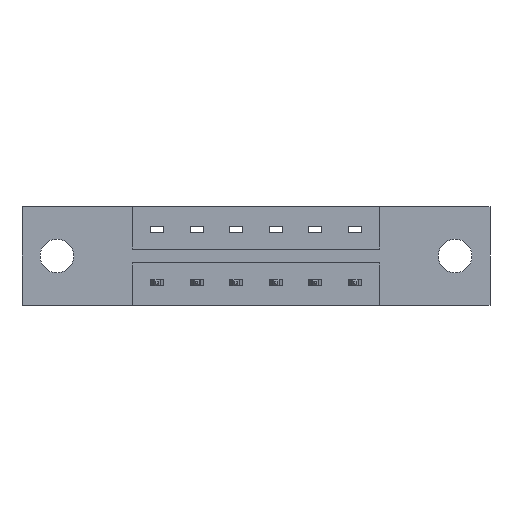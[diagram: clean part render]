
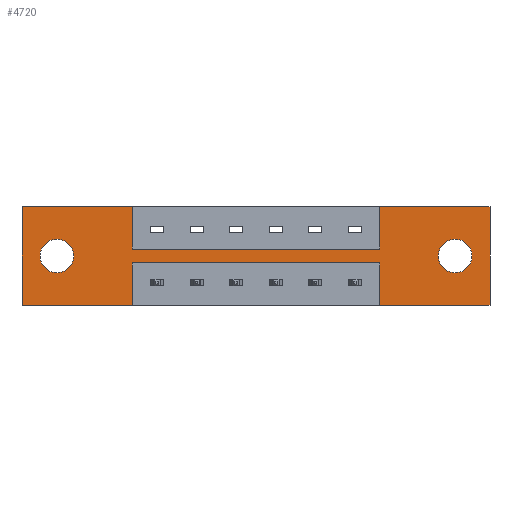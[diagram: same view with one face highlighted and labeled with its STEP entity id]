
A CAD part, front view. The second image highlights one B-rep face of the part: STEP entity #4720.
In plain terms, the highlighted planar face has unit normal (0, -1, 0).
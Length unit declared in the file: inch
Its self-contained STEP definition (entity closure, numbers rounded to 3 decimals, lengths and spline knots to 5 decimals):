
#126 = VERTEX_POINT ( 'NONE', #2826 ) ;
#157 = LINE ( 'NONE', #3902, #3286 ) ;
#171 = VECTOR ( 'NONE', #5851, 39.37008 ) ;
#455 = VECTOR ( 'NONE', #1524, 39.37008 ) ;
#487 = VERTEX_POINT ( 'NONE', #7712 ) ;
#570 = VECTOR ( 'NONE', #8237, 39.37008 ) ;
#605 = EDGE_CURVE ( 'NONE', #5778, #6451, #2992, .T. ) ;
#621 = CARTESIAN_POINT ( 'NONE',  ( 1.6425, 0., -0.2515 ) ) ;
#674 = ORIENTED_EDGE ( 'NONE', *, *, #7294, .F. ) ;
#721 = EDGE_CURVE ( 'NONE', #6205, #6852, #7734, .T. ) ;
#841 = EDGE_LOOP ( 'NONE', ( #1278, #674, #7091, #7510, #3355, #1827, #4442, #4466, #1448, #4593, #5694, #3701 ) ) ;
#894 = CARTESIAN_POINT ( 'NONE',  ( 0.4175, 0., -0.214 ) ) ;
#957 = EDGE_LOOP ( 'NONE', ( #3068, #5114 ) ) ;
#968 = CIRCLE ( 'NONE', #5069, 0.064 ) ;
#1029 = DIRECTION ( 'NONE',  ( 0., 1., 0. ) ) ;
#1107 = CARTESIAN_POINT ( 'NONE',  ( 0., 0., 0. ) ) ;
#1278 = ORIENTED_EDGE ( 'NONE', *, *, #4836, .F. ) ;
#1393 = EDGE_CURVE ( 'NONE', #1395, #4899, #5000, .T. ) ;
#1395 = VERTEX_POINT ( 'NONE', #6975 ) ;
#1448 = ORIENTED_EDGE ( 'NONE', *, *, #605, .F. ) ;
#1524 = DIRECTION ( 'NONE',  ( 0., 0., -1. ) ) ;
#1671 = LINE ( 'NONE', #2417, #5581 ) ;
#1817 = EDGE_CURVE ( 'NONE', #5523, #2225, #3481, .T. ) ;
#1827 = ORIENTED_EDGE ( 'NONE', *, *, #7455, .F. ) ;
#1871 = LINE ( 'NONE', #5779, #5684 ) ;
#1901 = EDGE_CURVE ( 'NONE', #2188, #126, #1984, .T. ) ;
#1923 = DIRECTION ( 'NONE',  ( 0., 0., -1. ) ) ;
#1935 = AXIS2_PLACEMENT_3D ( 'NONE', #4803, #6666, #2813 ) ;
#1984 = LINE ( 'NONE', #894, #455 ) ;
#2065 = CARTESIAN_POINT ( 'NONE',  ( 0.1325, 0., -0.2515 ) ) ;
#2150 = VERTEX_POINT ( 'NONE', #5043 ) ;
#2188 = VERTEX_POINT ( 'NONE', #6986 ) ;
#2211 = LINE ( 'NONE', #7557, #3015 ) ;
#2221 = CARTESIAN_POINT ( 'NONE',  ( 0.4175, 0., -0.161 ) ) ;
#2224 = CARTESIAN_POINT ( 'NONE',  ( 0.1325, 0., -0.1875 ) ) ;
#2225 = VERTEX_POINT ( 'NONE', #621 ) ;
#2317 = CARTESIAN_POINT ( 'NONE',  ( 0., 0., -0.375 ) ) ;
#2417 = CARTESIAN_POINT ( 'NONE',  ( 0.4175, 0., -0.214 ) ) ;
#2535 = AXIS2_PLACEMENT_3D ( 'NONE', #2224, #6041, #4019 ) ;
#2573 = VECTOR ( 'NONE', #5951, 39.37008 ) ;
#2580 = CARTESIAN_POINT ( 'NONE',  ( 0., 0., 0. ) ) ;
#2626 = LINE ( 'NONE', #5104, #5155 ) ;
#2667 = CARTESIAN_POINT ( 'NONE',  ( 1.3575, 0., -0.214 ) ) ;
#2702 = EDGE_CURVE ( 'NONE', #5014, #1395, #4282, .T. ) ;
#2813 = DIRECTION ( 'NONE',  ( 0., 0., -1. ) ) ;
#2826 = CARTESIAN_POINT ( 'NONE',  ( 0.4175, 0., -0.375 ) ) ;
#2886 = VECTOR ( 'NONE', #4833, 39.37008 ) ;
#2893 = CARTESIAN_POINT ( 'NONE',  ( 0.4175, 0., -0.161 ) ) ;
#2992 = LINE ( 'NONE', #4559, #171 ) ;
#3015 = VECTOR ( 'NONE', #3689, 39.37008 ) ;
#3050 = DIRECTION ( 'NONE',  ( -1., 0., 0. ) ) ;
#3068 = ORIENTED_EDGE ( 'NONE', *, *, #7592, .T. ) ;
#3094 = EDGE_CURVE ( 'NONE', #487, #4191, #6080, .T. ) ;
#3184 = DIRECTION ( 'NONE',  ( 0., 1., 0. ) ) ;
#3195 = ORIENTED_EDGE ( 'NONE', *, *, #1817, .T. ) ;
#3244 = CARTESIAN_POINT ( 'NONE',  ( 0.4175, 0., -0.161 ) ) ;
#3286 = VECTOR ( 'NONE', #6563, 39.37008 ) ;
#3355 = ORIENTED_EDGE ( 'NONE', *, *, #2702, .F. ) ;
#3417 = CARTESIAN_POINT ( 'NONE',  ( 1.3575, 0., -0.161 ) ) ;
#3471 = ORIENTED_EDGE ( 'NONE', *, *, #5888, .T. ) ;
#3481 = CIRCLE ( 'NONE', #1935, 0.064 ) ;
#3689 = DIRECTION ( 'NONE',  ( 0., 0., -1. ) ) ;
#3701 = ORIENTED_EDGE ( 'NONE', *, *, #7673, .F. ) ;
#3710 = AXIS2_PLACEMENT_3D ( 'NONE', #4911, #3184, #1923 ) ;
#3902 = CARTESIAN_POINT ( 'NONE',  ( 0., 0., -0.375 ) ) ;
#3934 = FACE_BOUND ( 'NONE', #957, .T. ) ;
#3955 = DIRECTION ( 'NONE',  ( -1., 0., 0. ) ) ;
#4019 = DIRECTION ( 'NONE',  ( 0., 0., 1. ) ) ;
#4191 = VERTEX_POINT ( 'NONE', #2221 ) ;
#4211 = CARTESIAN_POINT ( 'NONE',  ( 1.3575, 0., -0.375 ) ) ;
#4249 = DIRECTION ( 'NONE',  ( 0., -1., 0. ) ) ;
#4282 = LINE ( 'NONE', #3417, #2573 ) ;
#4351 = AXIS2_PLACEMENT_3D ( 'NONE', #2317, #4249, #8042 ) ;
#4366 = VECTOR ( 'NONE', #5685, 39.37008 ) ;
#4442 = ORIENTED_EDGE ( 'NONE', *, *, #3094, .F. ) ;
#4466 = ORIENTED_EDGE ( 'NONE', *, *, #4552, .F. ) ;
#4474 = DIRECTION ( 'NONE',  ( 0., 0., 1. ) ) ;
#4491 = LINE ( 'NONE', #2893, #2886 ) ;
#4521 = DIRECTION ( 'NONE',  ( 1., 0., 0. ) ) ;
#4552 = EDGE_CURVE ( 'NONE', #6451, #487, #7366, .T. ) ;
#4559 = CARTESIAN_POINT ( 'NONE',  ( 0., 0., 0. ) ) ;
#4593 = ORIENTED_EDGE ( 'NONE', *, *, #7313, .F. ) ;
#4706 = CARTESIAN_POINT ( 'NONE',  ( 0.1325, 0., -0.1235 ) ) ;
#4720 = ADVANCED_FACE ( 'NONE', ( #7069, #3934, #5359 ), #6132, .T. ) ;
#4727 = CARTESIAN_POINT ( 'NONE',  ( 1.6425, 0., -0.1235 ) ) ;
#4803 = CARTESIAN_POINT ( 'NONE',  ( 1.6425, 0., -0.1875 ) ) ;
#4833 = DIRECTION ( 'NONE',  ( 1., 0., 0. ) ) ;
#4836 = EDGE_CURVE ( 'NONE', #5768, #5450, #2626, .T. ) ;
#4899 = VERTEX_POINT ( 'NONE', #5167 ) ;
#4911 = CARTESIAN_POINT ( 'NONE',  ( 1.6425, 0., -0.1875 ) ) ;
#5000 = LINE ( 'NONE', #7517, #570 ) ;
#5014 = VERTEX_POINT ( 'NONE', #7264 ) ;
#5043 = CARTESIAN_POINT ( 'NONE',  ( 1.775, 0., -0.375 ) ) ;
#5069 = AXIS2_PLACEMENT_3D ( 'NONE', #6210, #1029, #6867 ) ;
#5104 = CARTESIAN_POINT ( 'NONE',  ( 1.3575, 0., -0.214 ) ) ;
#5114 = ORIENTED_EDGE ( 'NONE', *, *, #721, .T. ) ;
#5155 = VECTOR ( 'NONE', #4474, 39.37008 ) ;
#5167 = CARTESIAN_POINT ( 'NONE',  ( 1.775, 0., 0. ) ) ;
#5359 = FACE_OUTER_BOUND ( 'NONE', #841, .T. ) ;
#5450 = VERTEX_POINT ( 'NONE', #2667 ) ;
#5523 = VERTEX_POINT ( 'NONE', #4727 ) ;
#5581 = VECTOR ( 'NONE', #3050, 39.37008 ) ;
#5684 = VECTOR ( 'NONE', #3955, 39.37008 ) ;
#5685 = DIRECTION ( 'NONE',  ( 0., 0., -1. ) ) ;
#5694 = ORIENTED_EDGE ( 'NONE', *, *, #1901, .F. ) ;
#5768 = VERTEX_POINT ( 'NONE', #4211 ) ;
#5778 = VERTEX_POINT ( 'NONE', #7452 ) ;
#5779 = CARTESIAN_POINT ( 'NONE',  ( 0., 0., -0.375 ) ) ;
#5784 = EDGE_CURVE ( 'NONE', #4899, #2150, #2211, .T. ) ;
#5851 = DIRECTION ( 'NONE',  ( 0., 0., 1. ) ) ;
#5888 = EDGE_CURVE ( 'NONE', #2225, #5523, #7146, .T. ) ;
#5951 = DIRECTION ( 'NONE',  ( 0., 0., 1. ) ) ;
#6041 = DIRECTION ( 'NONE',  ( 0., 1., 0. ) ) ;
#6080 = LINE ( 'NONE', #3244, #4366 ) ;
#6132 = PLANE ( 'NONE',  #4351 ) ;
#6205 = VERTEX_POINT ( 'NONE', #2065 ) ;
#6210 = CARTESIAN_POINT ( 'NONE',  ( 0.1325, 0., -0.1875 ) ) ;
#6451 = VERTEX_POINT ( 'NONE', #1107 ) ;
#6563 = DIRECTION ( 'NONE',  ( -1., 0., 0. ) ) ;
#6666 = DIRECTION ( 'NONE',  ( 0., 1., 0. ) ) ;
#6668 = VECTOR ( 'NONE', #4521, 39.37008 ) ;
#6852 = VERTEX_POINT ( 'NONE', #4706 ) ;
#6867 = DIRECTION ( 'NONE',  ( 0., 0., 1. ) ) ;
#6880 = EDGE_LOOP ( 'NONE', ( #3195, #3471 ) ) ;
#6975 = CARTESIAN_POINT ( 'NONE',  ( 1.3575, 0., 0. ) ) ;
#6986 = CARTESIAN_POINT ( 'NONE',  ( 0.4175, 0., -0.214 ) ) ;
#7069 = FACE_BOUND ( 'NONE', #6880, .T. ) ;
#7091 = ORIENTED_EDGE ( 'NONE', *, *, #5784, .F. ) ;
#7146 = CIRCLE ( 'NONE', #3710, 0.064 ) ;
#7264 = CARTESIAN_POINT ( 'NONE',  ( 1.3575, 0., -0.161 ) ) ;
#7294 = EDGE_CURVE ( 'NONE', #2150, #5768, #157, .T. ) ;
#7313 = EDGE_CURVE ( 'NONE', #126, #5778, #1871, .T. ) ;
#7366 = LINE ( 'NONE', #2580, #6668 ) ;
#7452 = CARTESIAN_POINT ( 'NONE',  ( 0., 0., -0.375 ) ) ;
#7455 = EDGE_CURVE ( 'NONE', #4191, #5014, #4491, .T. ) ;
#7510 = ORIENTED_EDGE ( 'NONE', *, *, #1393, .F. ) ;
#7517 = CARTESIAN_POINT ( 'NONE',  ( 0., 0., 0. ) ) ;
#7557 = CARTESIAN_POINT ( 'NONE',  ( 1.775, 0., 0. ) ) ;
#7592 = EDGE_CURVE ( 'NONE', #6852, #6205, #968, .T. ) ;
#7673 = EDGE_CURVE ( 'NONE', #5450, #2188, #1671, .T. ) ;
#7712 = CARTESIAN_POINT ( 'NONE',  ( 0.4175, 0., 0. ) ) ;
#7734 = CIRCLE ( 'NONE', #2535, 0.064 ) ;
#8042 = DIRECTION ( 'NONE',  ( 0., 0., -1. ) ) ;
#8237 = DIRECTION ( 'NONE',  ( 1., 0., 0. ) ) ;
